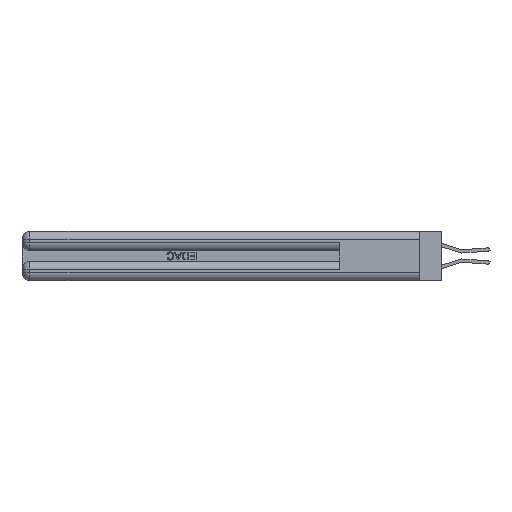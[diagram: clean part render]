
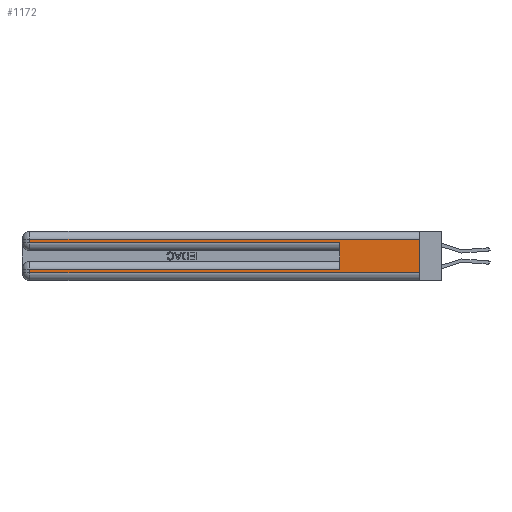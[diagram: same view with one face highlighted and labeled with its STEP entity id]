
A CAD part, left-side view. The second image highlights one B-rep face of the part: STEP entity #1172.
In plain terms, the highlighted planar face has unit normal (-1, 0, 0).
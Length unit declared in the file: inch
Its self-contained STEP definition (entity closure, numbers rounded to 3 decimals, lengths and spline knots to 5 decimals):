
#1172 = ADVANCED_FACE ( 'NONE', ( #8013 ), #27267, .F. ) ;
#1253 = CARTESIAN_POINT ( 'NONE',  ( 0., 0.6, 0.145 ) ) ;
#2085 = EDGE_LOOP ( 'NONE', ( #38853, #4896, #13252, #28228, #31392, #23280, #37446, #37925 ) ) ;
#2138 = LINE ( 'NONE', #4301, #12150 ) ;
#2280 = CARTESIAN_POINT ( 'NONE',  ( 0., 0., 0.285 ) ) ;
#2485 = LINE ( 'NONE', #9958, #15378 ) ;
#2711 = LINE ( 'NONE', #14187, #39599 ) ;
#3092 = VERTEX_POINT ( 'NONE', #28405 ) ;
#4301 = CARTESIAN_POINT ( 'NONE',  ( 0., 0., 0.06 ) ) ;
#4686 = LINE ( 'NONE', #2280, #19197 ) ;
#4896 = ORIENTED_EDGE ( 'NONE', *, *, #41557, .T. ) ;
#6631 = LINE ( 'NONE', #12395, #34058 ) ;
#7169 = CARTESIAN_POINT ( 'NONE',  ( 0., 2.94, 0.285 ) ) ;
#8013 = FACE_OUTER_BOUND ( 'NONE', #2085, .T. ) ;
#9958 = CARTESIAN_POINT ( 'NONE',  ( 0., 2.94, 0.37 ) ) ;
#10132 = DIRECTION ( 'NONE',  ( 1., 0., 0. ) ) ;
#10960 = DIRECTION ( 'NONE',  ( 0., 0., -1. ) ) ;
#12150 = VECTOR ( 'NONE', #36611, 39.37008 ) ;
#12395 = CARTESIAN_POINT ( 'NONE',  ( 0., 0., 0.31 ) ) ;
#13252 = ORIENTED_EDGE ( 'NONE', *, *, #31046, .T. ) ;
#13264 = CARTESIAN_POINT ( 'NONE',  ( 0., 0., 0.37 ) ) ;
#14187 = CARTESIAN_POINT ( 'NONE',  ( 0., 0., 0.085 ) ) ;
#15378 = VECTOR ( 'NONE', #41839, 39.37008 ) ;
#15725 = VECTOR ( 'NONE', #10960, 39.37008 ) ;
#16209 = VECTOR ( 'NONE', #38674, 39.37008 ) ;
#16343 = CARTESIAN_POINT ( 'NONE',  ( 0., 0.6, 0.085 ) ) ;
#17539 = CARTESIAN_POINT ( 'NONE',  ( 0., 2.94, 0.37 ) ) ;
#17796 = EDGE_CURVE ( 'NONE', #32731, #39064, #2711, .T. ) ;
#19197 = VECTOR ( 'NONE', #27476, 39.37008 ) ;
#19742 = EDGE_CURVE ( 'NONE', #32731, #32490, #33938, .T. ) ;
#22145 = CARTESIAN_POINT ( 'NONE',  ( 0., 0., 0.06 ) ) ;
#23280 = ORIENTED_EDGE ( 'NONE', *, *, #17796, .T. ) ;
#23319 = AXIS2_PLACEMENT_3D ( 'NONE', #13264, #10132, #34542 ) ;
#23524 = LINE ( 'NONE', #27948, #16209 ) ;
#25957 = VERTEX_POINT ( 'NONE', #7169 ) ;
#26946 = CARTESIAN_POINT ( 'NONE',  ( 0., 0., 0.31 ) ) ;
#27267 = PLANE ( 'NONE',  #23319 ) ;
#27476 = DIRECTION ( 'NONE',  ( 0., -1., 0. ) ) ;
#27480 = LINE ( 'NONE', #17539, #15725 ) ;
#27948 = CARTESIAN_POINT ( 'NONE',  ( 0., 0., 0.37 ) ) ;
#28228 = ORIENTED_EDGE ( 'NONE', *, *, #45514, .T. ) ;
#28405 = CARTESIAN_POINT ( 'NONE',  ( 0., 2.94, 0.06 ) ) ;
#29327 = VERTEX_POINT ( 'NONE', #22145 ) ;
#30691 = VERTEX_POINT ( 'NONE', #44267 ) ;
#31046 = EDGE_CURVE ( 'NONE', #30691, #25957, #27480, .T. ) ;
#31392 = ORIENTED_EDGE ( 'NONE', *, *, #19742, .F. ) ;
#32490 = VERTEX_POINT ( 'NONE', #36510 ) ;
#32731 = VERTEX_POINT ( 'NONE', #16343 ) ;
#33561 = DIRECTION ( 'NONE',  ( 0., 1., 0. ) ) ;
#33801 = EDGE_CURVE ( 'NONE', #43589, #29327, #23524, .T. ) ;
#33938 = LINE ( 'NONE', #1253, #46079 ) ;
#34058 = VECTOR ( 'NONE', #33561, 39.37008 ) ;
#34542 = DIRECTION ( 'NONE',  ( 0., 0., -1. ) ) ;
#36510 = CARTESIAN_POINT ( 'NONE',  ( 0., 0.6, 0.285 ) ) ;
#36611 = DIRECTION ( 'NONE',  ( 0., -1., 0. ) ) ;
#37446 = ORIENTED_EDGE ( 'NONE', *, *, #43766, .T. ) ;
#37925 = ORIENTED_EDGE ( 'NONE', *, *, #42005, .T. ) ;
#38674 = DIRECTION ( 'NONE',  ( 0., 0., -1. ) ) ;
#38853 = ORIENTED_EDGE ( 'NONE', *, *, #33801, .F. ) ;
#39064 = VERTEX_POINT ( 'NONE', #43427 ) ;
#39599 = VECTOR ( 'NONE', #42451, 39.37008 ) ;
#40625 = DIRECTION ( 'NONE',  ( 0., 0., 1. ) ) ;
#41557 = EDGE_CURVE ( 'NONE', #43589, #30691, #6631, .T. ) ;
#41839 = DIRECTION ( 'NONE',  ( 0., 0., -1. ) ) ;
#42005 = EDGE_CURVE ( 'NONE', #3092, #29327, #2138, .T. ) ;
#42451 = DIRECTION ( 'NONE',  ( 0., 1., 0. ) ) ;
#43427 = CARTESIAN_POINT ( 'NONE',  ( 0., 2.94, 0.085 ) ) ;
#43589 = VERTEX_POINT ( 'NONE', #26946 ) ;
#43766 = EDGE_CURVE ( 'NONE', #39064, #3092, #2485, .T. ) ;
#44267 = CARTESIAN_POINT ( 'NONE',  ( 0., 2.94, 0.31 ) ) ;
#45514 = EDGE_CURVE ( 'NONE', #25957, #32490, #4686, .T. ) ;
#46079 = VECTOR ( 'NONE', #40625, 39.37008 ) ;
